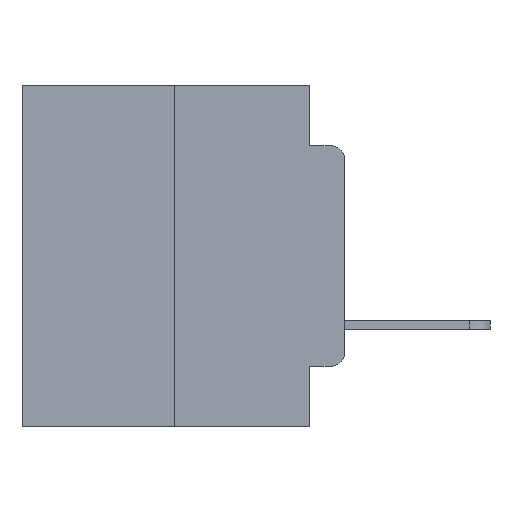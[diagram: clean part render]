
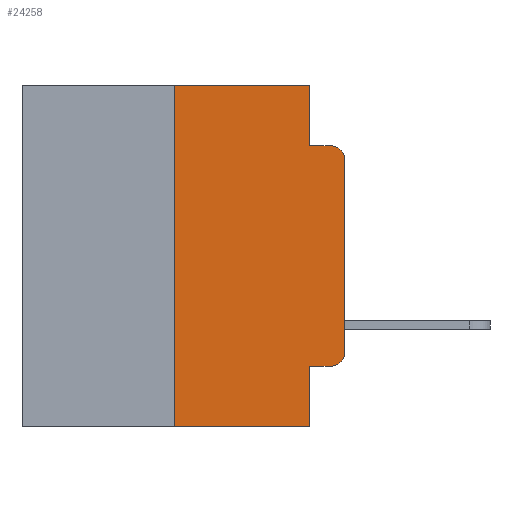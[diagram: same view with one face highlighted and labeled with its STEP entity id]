
A CAD part, left-side view. The second image highlights one B-rep face of the part: STEP entity #24258.
In plain terms, the highlighted planar face has unit normal (-1, 0, 0).
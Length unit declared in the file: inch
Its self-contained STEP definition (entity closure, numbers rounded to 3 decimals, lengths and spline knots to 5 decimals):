
#690 = CARTESIAN_POINT ( 'NONE',  ( 0., 0.02, -0.4115 ) ) ;
#808 = VECTOR ( 'NONE', #2939, 39.37008 ) ;
#950 = CARTESIAN_POINT ( 'NONE',  ( 0., 0.02, -0.1085 ) ) ;
#1172 = DIRECTION ( 'NONE',  ( 0., 0., -1. ) ) ;
#1174 = CARTESIAN_POINT ( 'NONE',  ( 0., 0., -0.1085 ) ) ;
#1205 = DIRECTION ( 'NONE',  ( -1., 0., 0. ) ) ;
#1360 = CARTESIAN_POINT ( 'NONE',  ( 0., 0.051, 0. ) ) ;
#1665 = CARTESIAN_POINT ( 'NONE',  ( 0., 0.02, -0.0885 ) ) ;
#1949 = VECTOR ( 'NONE', #14006, 39.37008 ) ;
#2260 = CARTESIAN_POINT ( 'NONE',  ( 0., 0.051, -0.0885 ) ) ;
#2633 = VERTEX_POINT ( 'NONE', #1665 ) ;
#2699 = EDGE_CURVE ( 'NONE', #5484, #2633, #22149, .T. ) ;
#2731 = VERTEX_POINT ( 'NONE', #690 ) ;
#2916 = LINE ( 'NONE', #1360, #23418 ) ;
#2939 = DIRECTION ( 'NONE',  ( 0., -1., 0. ) ) ;
#3269 = AXIS2_PLACEMENT_3D ( 'NONE', #22601, #10320, #24566 ) ;
#3473 = EDGE_CURVE ( 'NONE', #22644, #2731, #12836, .T. ) ;
#3801 = VECTOR ( 'NONE', #9451, 39.37008 ) ;
#4128 = EDGE_CURVE ( 'NONE', #7482, #2633, #11867, .T. ) ;
#4904 = EDGE_CURVE ( 'NONE', #2731, #25776, #12824, .T. ) ;
#5484 = VERTEX_POINT ( 'NONE', #1174 ) ;
#5547 = DIRECTION ( 'NONE',  ( 0., 0., -1. ) ) ;
#5732 = DIRECTION ( 'NONE',  ( 0., -1., 0. ) ) ;
#5887 = CARTESIAN_POINT ( 'NONE',  ( 0., 0.25, 0. ) ) ;
#6303 = CARTESIAN_POINT ( 'NONE',  ( 0., 0.473, 0. ) ) ;
#6597 = VERTEX_POINT ( 'NONE', #23405 ) ;
#7356 = VECTOR ( 'NONE', #5732, 39.37008 ) ;
#7482 = VERTEX_POINT ( 'NONE', #26245 ) ;
#8308 = DIRECTION ( 'NONE',  ( 0., -1., 0. ) ) ;
#8597 = EDGE_CURVE ( 'NONE', #6597, #11571, #14089, .T. ) ;
#8753 = ORIENTED_EDGE ( 'NONE', *, *, #3473, .T. ) ;
#8860 = ORIENTED_EDGE ( 'NONE', *, *, #4904, .T. ) ;
#8937 = LINE ( 'NONE', #11997, #19269 ) ;
#9060 = ORIENTED_EDGE ( 'NONE', *, *, #20478, .F. ) ;
#9451 = DIRECTION ( 'NONE',  ( 0., 0., 1. ) ) ;
#9664 = VECTOR ( 'NONE', #8308, 39.37008 ) ;
#9843 = CARTESIAN_POINT ( 'NONE',  ( 0., 0.473, -0.5 ) ) ;
#9881 = ORIENTED_EDGE ( 'NONE', *, *, #12801, .T. ) ;
#10155 = CARTESIAN_POINT ( 'NONE',  ( 0., 0.051, -0.5 ) ) ;
#10313 = LINE ( 'NONE', #6303, #9664 ) ;
#10320 = DIRECTION ( 'NONE',  ( 1., 0., 0. ) ) ;
#10330 = CARTESIAN_POINT ( 'NONE',  ( 0., 0.02, -0.3915 ) ) ;
#11266 = VERTEX_POINT ( 'NONE', #14671 ) ;
#11447 = LINE ( 'NONE', #21678, #21731 ) ;
#11568 = CARTESIAN_POINT ( 'NONE',  ( 0., 0.051, -0.4115 ) ) ;
#11571 = VERTEX_POINT ( 'NONE', #5887 ) ;
#11867 = LINE ( 'NONE', #2260, #808 ) ;
#11997 = CARTESIAN_POINT ( 'NONE',  ( 0., 0.051, 0. ) ) ;
#12235 = CARTESIAN_POINT ( 'NONE',  ( 0., 0.25, 0. ) ) ;
#12801 = EDGE_CURVE ( 'NONE', #6597, #18525, #12930, .T. ) ;
#12824 = CIRCLE ( 'NONE', #17747, 0.02 ) ;
#12836 = LINE ( 'NONE', #24534, #7356 ) ;
#12930 = LINE ( 'NONE', #9843, #1949 ) ;
#14006 = DIRECTION ( 'NONE',  ( 0., -1., 0. ) ) ;
#14089 = LINE ( 'NONE', #12235, #3801 ) ;
#14093 = DIRECTION ( 'NONE',  ( 0., 0., -1. ) ) ;
#14671 = CARTESIAN_POINT ( 'NONE',  ( 0., 0.051, 0. ) ) ;
#14795 = ORIENTED_EDGE ( 'NONE', *, *, #8597, .F. ) ;
#16249 = ORIENTED_EDGE ( 'NONE', *, *, #25092, .T. ) ;
#16656 = ORIENTED_EDGE ( 'NONE', *, *, #2699, .T. ) ;
#16836 = DIRECTION ( 'NONE',  ( 0., 0., -1. ) ) ;
#16841 = FACE_OUTER_BOUND ( 'NONE', #18793, .T. ) ;
#16863 = DIRECTION ( 'NONE',  ( -1., 0., 0. ) ) ;
#17422 = ORIENTED_EDGE ( 'NONE', *, *, #4128, .F. ) ;
#17684 = ORIENTED_EDGE ( 'NONE', *, *, #19263, .F. ) ;
#17747 = AXIS2_PLACEMENT_3D ( 'NONE', #10330, #16863, #16836 ) ;
#18211 = ORIENTED_EDGE ( 'NONE', *, *, #19185, .F. ) ;
#18525 = VERTEX_POINT ( 'NONE', #10155 ) ;
#18793 = EDGE_LOOP ( 'NONE', ( #16249, #16656, #17422, #17684, #18211, #14795, #9881, #9060, #8753, #8860 ) ) ;
#19185 = EDGE_CURVE ( 'NONE', #11571, #11266, #10313, .T. ) ;
#19263 = EDGE_CURVE ( 'NONE', #11266, #7482, #2916, .T. ) ;
#19269 = VECTOR ( 'NONE', #14093, 39.37008 ) ;
#20478 = EDGE_CURVE ( 'NONE', #22644, #18525, #8937, .T. ) ;
#20545 = PLANE ( 'NONE',  #3269 ) ;
#21678 = CARTESIAN_POINT ( 'NONE',  ( 0., 0., 0. ) ) ;
#21731 = VECTOR ( 'NONE', #23656, 39.37008 ) ;
#22149 = CIRCLE ( 'NONE', #24626, 0.02 ) ;
#22601 = CARTESIAN_POINT ( 'NONE',  ( 0., 0.473, 0. ) ) ;
#22644 = VERTEX_POINT ( 'NONE', #11568 ) ;
#23405 = CARTESIAN_POINT ( 'NONE',  ( 0., 0.25, -0.5 ) ) ;
#23418 = VECTOR ( 'NONE', #5547, 39.37008 ) ;
#23656 = DIRECTION ( 'NONE',  ( 0., 0., 1. ) ) ;
#23804 = CARTESIAN_POINT ( 'NONE',  ( 0., 0., -0.3915 ) ) ;
#24258 = ADVANCED_FACE ( 'NONE', ( #16841 ), #20545, .F. ) ;
#24534 = CARTESIAN_POINT ( 'NONE',  ( 0., 0.051, -0.4115 ) ) ;
#24566 = DIRECTION ( 'NONE',  ( 0., 0., -1. ) ) ;
#24626 = AXIS2_PLACEMENT_3D ( 'NONE', #950, #1205, #1172 ) ;
#25092 = EDGE_CURVE ( 'NONE', #25776, #5484, #11447, .T. ) ;
#25776 = VERTEX_POINT ( 'NONE', #23804 ) ;
#26245 = CARTESIAN_POINT ( 'NONE',  ( 0., 0.051, -0.0885 ) ) ;
